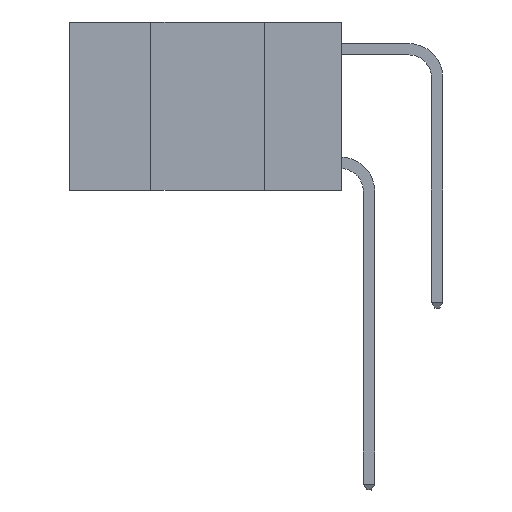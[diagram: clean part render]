
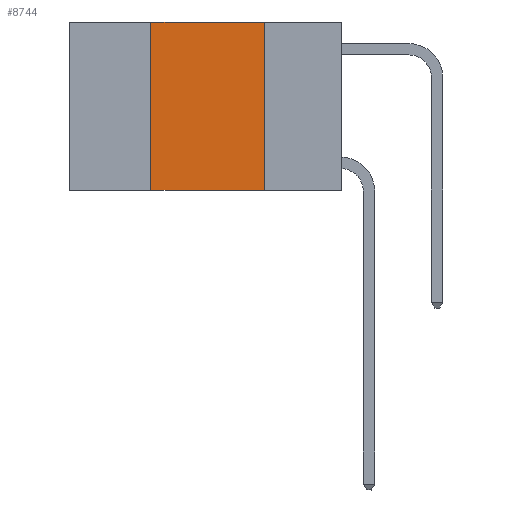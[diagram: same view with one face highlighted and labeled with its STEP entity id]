
A CAD part, left-side view. The second image highlights one B-rep face of the part: STEP entity #8744.
In plain terms, the highlighted planar face has unit normal (-1, 0, 0).
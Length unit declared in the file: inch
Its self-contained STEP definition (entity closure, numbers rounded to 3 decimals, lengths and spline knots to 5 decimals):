
#545 = VERTEX_POINT ( 'NONE', #6721 ) ;
#611 = CARTESIAN_POINT ( 'NONE',  ( 0., 0.17, 0. ) ) ;
#787 = CARTESIAN_POINT ( 'NONE',  ( 0., 0.6, 0. ) ) ;
#1302 = ORIENTED_EDGE ( 'NONE', *, *, #4941, .T. ) ;
#2973 = VECTOR ( 'NONE', #10556, 39.37008 ) ;
#3676 = CARTESIAN_POINT ( 'NONE',  ( 0., 0.42, 0. ) ) ;
#3862 = CARTESIAN_POINT ( 'NONE',  ( 0., 0.6, -0.37 ) ) ;
#4941 = EDGE_CURVE ( 'NONE', #5224, #7196, #23192, .T. ) ;
#5224 = VERTEX_POINT ( 'NONE', #17434 ) ;
#6504 = LINE ( 'NONE', #611, #18387 ) ;
#6721 = CARTESIAN_POINT ( 'NONE',  ( 0., 0.17, 0. ) ) ;
#7196 = VERTEX_POINT ( 'NONE', #14888 ) ;
#8541 = EDGE_CURVE ( 'NONE', #22617, #545, #21224, .T. ) ;
#8744 = ADVANCED_FACE ( 'NONE', ( #25075 ), #18286, .F. ) ;
#9406 = ORIENTED_EDGE ( 'NONE', *, *, #20817, .F. ) ;
#10556 = DIRECTION ( 'NONE',  ( 0., -1., 0. ) ) ;
#11615 = DIRECTION ( 'NONE',  ( 1., 0., 0. ) ) ;
#12786 = DIRECTION ( 'NONE',  ( 0., 0., -1. ) ) ;
#12988 = ORIENTED_EDGE ( 'NONE', *, *, #8541, .F. ) ;
#13319 = CARTESIAN_POINT ( 'NONE',  ( 0., 0.6, 0. ) ) ;
#13597 = EDGE_CURVE ( 'NONE', #545, #7196, #6504, .T. ) ;
#13933 = EDGE_LOOP ( 'NONE', ( #16878, #12988, #9406, #1302 ) ) ;
#14888 = CARTESIAN_POINT ( 'NONE',  ( 0., 0.17, -0.37 ) ) ;
#15209 = VECTOR ( 'NONE', #17614, 39.37008 ) ;
#16483 = CARTESIAN_POINT ( 'NONE',  ( 0., 0.42, 0. ) ) ;
#16878 = ORIENTED_EDGE ( 'NONE', *, *, #13597, .F. ) ;
#17434 = CARTESIAN_POINT ( 'NONE',  ( 0., 0.42, -0.37 ) ) ;
#17614 = DIRECTION ( 'NONE',  ( 0., -1., 0. ) ) ;
#18286 = PLANE ( 'NONE',  #25545 ) ;
#18387 = VECTOR ( 'NONE', #25179, 39.37008 ) ;
#20817 = EDGE_CURVE ( 'NONE', #5224, #22617, #26305, .T. ) ;
#21224 = LINE ( 'NONE', #13319, #15209 ) ;
#21345 = DIRECTION ( 'NONE',  ( 0., 0., 1. ) ) ;
#22617 = VERTEX_POINT ( 'NONE', #16483 ) ;
#23192 = LINE ( 'NONE', #3862, #2973 ) ;
#25075 = FACE_OUTER_BOUND ( 'NONE', #13933, .T. ) ;
#25179 = DIRECTION ( 'NONE',  ( 0., 0., -1. ) ) ;
#25545 = AXIS2_PLACEMENT_3D ( 'NONE', #787, #11615, #12786 ) ;
#26305 = LINE ( 'NONE', #3676, #27006 ) ;
#27006 = VECTOR ( 'NONE', #21345, 39.37008 ) ;
